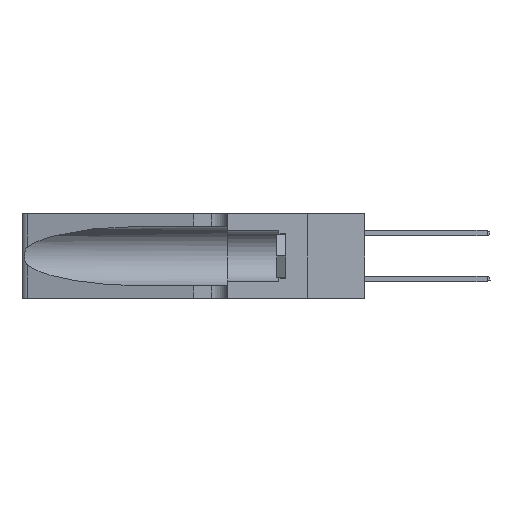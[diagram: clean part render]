
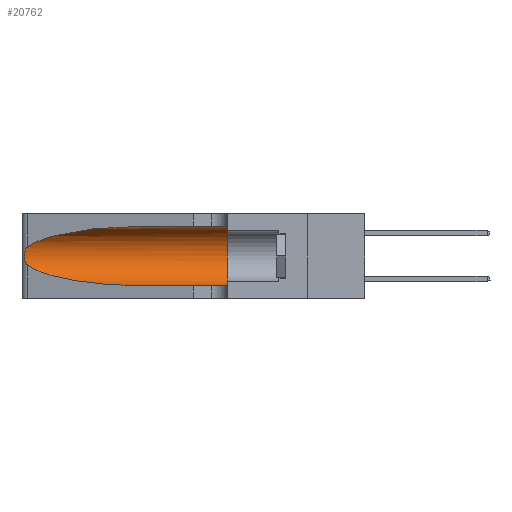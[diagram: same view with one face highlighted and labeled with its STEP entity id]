
A CAD part, left-side view. The second image highlights one B-rep face of the part: STEP entity #20762.
In plain terms, the highlighted cylindrical face has radius 3.308 mm (diameter 6.617 mm), a partial arc.
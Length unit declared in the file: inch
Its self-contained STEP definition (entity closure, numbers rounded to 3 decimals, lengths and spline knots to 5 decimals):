
#204 = VERTEX_POINT ( 'NONE', #39173 ) ;
#290 = B_SPLINE_CURVE_WITH_KNOTS ( 'NONE', 3,
 ( #35375, #12395, #38669, #19070, #41984, #22379, #2303, #25674, #5705, #28975, #9122, #32245, #12533, #35515 ),
 .UNSPECIFIED., .F., .F.,
 ( 4, 2, 2, 2, 2, 2, 4 ),
 ( 0., 0.00027, 0.00053, 0.00107, 0.0016, 0.00187, 0.00214 ),
 .UNSPECIFIED. ) ;
#609 = VECTOR ( 'NONE', #30066, 39.37008 ) ;
#2303 = CARTESIAN_POINT ( 'NONE',  ( 0.26075, 1.23896, 0.19203 ) ) ;
#2509 = EDGE_CURVE ( 'NONE', #33887, #40379, #37000, .T. ) ;
#2554 = AXIS2_PLACEMENT_3D ( 'NONE', #23767, #40203, #17288 ) ;
#3465 = CARTESIAN_POINT ( 'NONE',  ( 0.1305, 0.72297, 0.05475 ) ) ;
#4568 = FACE_OUTER_BOUND ( 'NONE', #5658, .T. ) ;
#5305 = ORIENTED_EDGE ( 'NONE', *, *, #25739, .F. ) ;
#5658 = EDGE_LOOP ( 'NONE', ( #38906, #16062, #19936, #40444, #5305, #41795 ) ) ;
#5705 = CARTESIAN_POINT ( 'NONE',  ( 0.26017, 1.23833, 0.17102 ) ) ;
#6023 = DIRECTION ( 'NONE',  ( 0., -1., 0. ) ) ;
#6837 = CARTESIAN_POINT ( 'NONE',  ( 0.1305, 1.61858, 0.31525 ) ) ;
#7206 = EDGE_CURVE ( 'NONE', #204, #14950, #290, .T. ) ;
#9122 = CARTESIAN_POINT ( 'NONE',  ( 0.25789, 1.23486, 0.15765 ) ) ;
#9911 = CARTESIAN_POINT ( 'NONE',  ( 0.1305, 0.35, 0.185 ) ) ;
#12395 = CARTESIAN_POINT ( 'NONE',  ( 0.25555, 1.22994, 0.2215 ) ) ;
#12533 = CARTESIAN_POINT ( 'NONE',  ( 0.25555, 1.22993, 0.14849 ) ) ;
#12830 = CARTESIAN_POINT ( 'NONE',  ( 0.1305, 1.61858, 0.05475 ) ) ;
#13291 = DIRECTION ( 'NONE',  ( 0., 0., 1. ) ) ;
#13435 = CARTESIAN_POINT ( 'NONE',  ( 0.1305, 0.72297, 0.31525 ) ) ;
#14106 = EDGE_CURVE ( 'NONE', #33887, #204, #35723, .T. ) ;
#14950 = VERTEX_POINT ( 'NONE', #27372 ) ;
#15201 = VECTOR ( 'NONE', #6023, 39.37008 ) ;
#16062 = ORIENTED_EDGE ( 'NONE', *, *, #7206, .T. ) ;
#16771 = CARTESIAN_POINT ( 'NONE',  ( 0.18966, 0.96281, 0.31525 ) ) ;
#16856 = CARTESIAN_POINT ( 'NONE',  ( 0.2373, 1.15595, 0.08982 ) ) ;
#17288 = DIRECTION ( 'NONE',  ( 0., 0., -1. ) ) ;
#17977 = CARTESIAN_POINT ( 'NONE',  ( 0.1305, 0.35, 0.05475 ) ) ;
#19070 = CARTESIAN_POINT ( 'NONE',  ( 0.25787, 1.23484, 0.2124 ) ) ;
#19936 = ORIENTED_EDGE ( 'NONE', *, *, #22613, .T. ) ;
#20182 = CARTESIAN_POINT ( 'NONE',  ( 0.25487, 1.22718, 0.14631 ) ) ;
#20762 = ADVANCED_FACE ( 'NONE', ( #4568 ), #30075, .F. ) ;
#22379 = CARTESIAN_POINT ( 'NONE',  ( 0.26018, 1.23835, 0.19895 ) ) ;
#22613 = EDGE_CURVE ( 'NONE', #14950, #29312, #32595, .T. ) ;
#23412 = CARTESIAN_POINT ( 'NONE',  ( 0.25487, 1.22718, 0.22369 ) ) ;
#23494 = CARTESIAN_POINT ( 'NONE',  ( 0.18966, 0.96281, 0.05475 ) ) ;
#23767 = CARTESIAN_POINT ( 'NONE',  ( 0.1305, 1.61858, 0.185 ) ) ;
#24002 = LINE ( 'NONE', #12830, #15201 ) ;
#24468 = CARTESIAN_POINT ( 'NONE',  ( 0.1305, 0.72297, 0.05475 ) ) ;
#25674 = CARTESIAN_POINT ( 'NONE',  ( 0.26075, 1.23896, 0.178 ) ) ;
#25739 = EDGE_CURVE ( 'NONE', #40379, #31313, #37006, .T. ) ;
#27372 = CARTESIAN_POINT ( 'NONE',  ( 0.25487, 1.22718, 0.14631 ) ) ;
#28975 = CARTESIAN_POINT ( 'NONE',  ( 0.25856, 1.23593, 0.16098 ) ) ;
#29312 = VERTEX_POINT ( 'NONE', #24468 ) ;
#30066 = DIRECTION ( 'NONE',  ( 0., -1., 0. ) ) ;
#30075 = CYLINDRICAL_SURFACE ( 'NONE', #2554, 0.13025 ) ;
#31313 = VERTEX_POINT ( 'NONE', #17977 ) ;
#32245 = CARTESIAN_POINT ( 'NONE',  ( 0.25639, 1.23186, 0.15144 ) ) ;
#32595 =( BOUNDED_CURVE ( )  B_SPLINE_CURVE ( 3, ( #20182, #16856, #23494, #3465 ),
 .UNSPECIFIED., .F., .F. ) 
 B_SPLINE_CURVE_WITH_KNOTS ( ( 4, 4 ),
 ( 3.44316, 4.71239 ),
 .UNSPECIFIED. ) 
 CURVE ( )  GEOMETRIC_REPRESENTATION_ITEM ( )  RATIONAL_B_SPLINE_CURVE ( ( 1., 0.87, 0.87, 1. ) ) 
 REPRESENTATION_ITEM ( '' )  );
#32994 = DIRECTION ( 'NONE',  ( 0., 1., 0. ) ) ;
#33848 = AXIS2_PLACEMENT_3D ( 'NONE', #9911, #32994, #13291 ) ;
#33887 = VERTEX_POINT ( 'NONE', #39751 ) ;
#33968 = CARTESIAN_POINT ( 'NONE',  ( 0.2373, 1.15595, 0.28018 ) ) ;
#35375 = CARTESIAN_POINT ( 'NONE',  ( 0.25487, 1.22718, 0.22369 ) ) ;
#35515 = CARTESIAN_POINT ( 'NONE',  ( 0.25487, 1.22718, 0.14631 ) ) ;
#35723 =( BOUNDED_CURVE ( )  B_SPLINE_CURVE ( 3, ( #13435, #16771, #33968, #23412 ),
 .UNSPECIFIED., .F., .F. ) 
 B_SPLINE_CURVE_WITH_KNOTS ( ( 4, 4 ),
 ( 1.5708, 2.84003 ),
 .UNSPECIFIED. ) 
 CURVE ( )  GEOMETRIC_REPRESENTATION_ITEM ( )  RATIONAL_B_SPLINE_CURVE ( ( 1., 0.87, 0.87, 1. ) ) 
 REPRESENTATION_ITEM ( '' )  );
#37000 = LINE ( 'NONE', #6837, #609 ) ;
#37006 = CIRCLE ( 'NONE', #33848, 0.13025 ) ;
#38669 = CARTESIAN_POINT ( 'NONE',  ( 0.25639, 1.23184, 0.21858 ) ) ;
#38906 = ORIENTED_EDGE ( 'NONE', *, *, #14106, .T. ) ;
#39173 = CARTESIAN_POINT ( 'NONE',  ( 0.25487, 1.22718, 0.22369 ) ) ;
#39223 = CARTESIAN_POINT ( 'NONE',  ( 0.1305, 0.35, 0.31525 ) ) ;
#39633 = EDGE_CURVE ( 'NONE', #29312, #31313, #24002, .T. ) ;
#39751 = CARTESIAN_POINT ( 'NONE',  ( 0.1305, 0.72297, 0.31525 ) ) ;
#40203 = DIRECTION ( 'NONE',  ( 0., -1., 0. ) ) ;
#40379 = VERTEX_POINT ( 'NONE', #39223 ) ;
#40444 = ORIENTED_EDGE ( 'NONE', *, *, #39633, .T. ) ;
#41795 = ORIENTED_EDGE ( 'NONE', *, *, #2509, .F. ) ;
#41984 = CARTESIAN_POINT ( 'NONE',  ( 0.25854, 1.2359, 0.20912 ) ) ;
